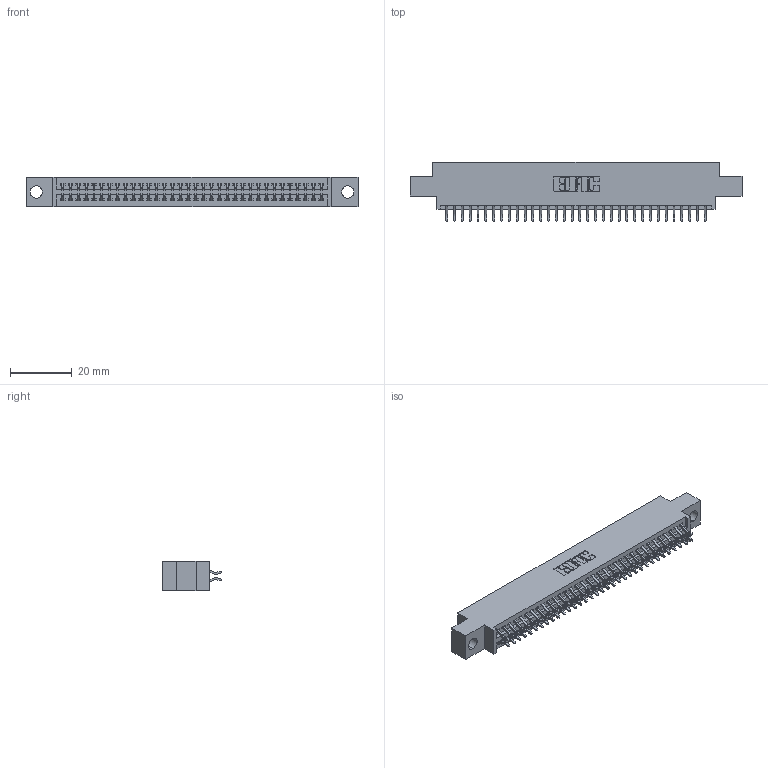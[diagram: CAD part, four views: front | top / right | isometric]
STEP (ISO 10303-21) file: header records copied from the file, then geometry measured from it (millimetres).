
FILE_DESCRIPTION (( 'STEP AP203' ), '1' );
FILE_NAME ('395-068-556-804.STEP', '2021-06-17T04:08:43', ( '' ), ( '' ), 'SwSTEP 2.0', 'SolidWorks 2020', '' );
FILE_SCHEMA (( 'CONFIG_CONTROL_DESIGN' ));
Length unit declared in the file: inch
Products named in the file (3): 395-068-556-804; 345 Part_0.170 Offset - 0.156 Dia-TI; 345-292-001_556 Tail
Assembly tree (69 placements, depth 2):
  395-068-556-804
    345 Part_0.170 Offset - 0.156 Dia-TI
    345-292-001_556 Tail  x68
Bounding box: 107.57 x 19.24 x 9.4 mm (x, y, z)
Volume: 10153.1 mm3; surface area: 14788.6 mm2
Topology: 69 solids, 69 shells, 3952 faces, 11745 edges, 7738 vertices
Faces by surface type: plane 2614, cylinder 1338
Entity records: 28525 total; most frequent: CARTESIAN_POINT 4810, ORIENTED_EDGE 4730, DIRECTION 4237, EDGE_CURVE 2365, VECTOR 2089, LINE 2089, VERTEX_POINT 1574, AXIS2_PLACEMENT_3D 1074
